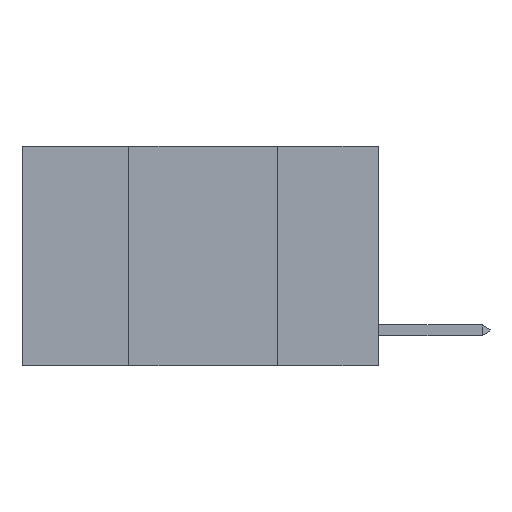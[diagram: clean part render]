
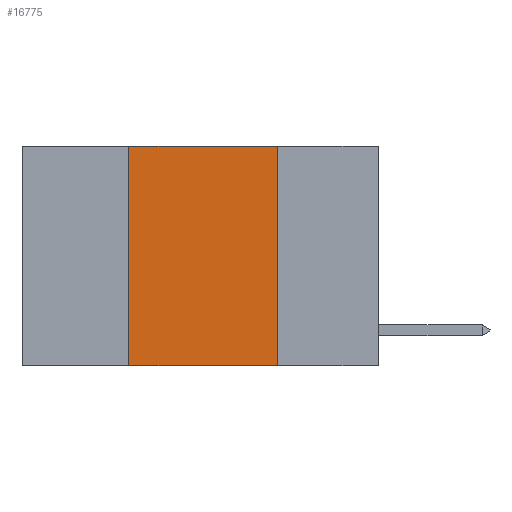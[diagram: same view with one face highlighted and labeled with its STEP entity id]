
A CAD part, left-side view. The second image highlights one B-rep face of the part: STEP entity #16775.
In plain terms, the highlighted planar face has unit normal (-1, 0, 0).
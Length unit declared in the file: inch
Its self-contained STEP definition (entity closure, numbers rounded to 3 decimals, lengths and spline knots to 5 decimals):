
#320 = ORIENTED_EDGE ( 'NONE', *, *, #9972, .T. ) ;
#625 = EDGE_CURVE ( 'NONE', #6422, #5239, #4161, .T. ) ;
#1381 = EDGE_CURVE ( 'NONE', #10255, #18290, #10004, .T. ) ;
#1623 = PLANE ( 'NONE',  #4414 ) ;
#2044 = DIRECTION ( 'NONE',  ( 0., -1., 0. ) ) ;
#2217 = CARTESIAN_POINT ( 'NONE',  ( 0., 0.17, 0. ) ) ;
#3463 = CARTESIAN_POINT ( 'NONE',  ( 0., 0.17, -0.37 ) ) ;
#3628 = CARTESIAN_POINT ( 'NONE',  ( 0., 0.6, -0.37 ) ) ;
#3800 = LINE ( 'NONE', #19191, #20383 ) ;
#4077 = ORIENTED_EDGE ( 'NONE', *, *, #1381, .F. ) ;
#4161 = LINE ( 'NONE', #2217, #12407 ) ;
#4414 = AXIS2_PLACEMENT_3D ( 'NONE', #5006, #17934, #8306 ) ;
#5006 = CARTESIAN_POINT ( 'NONE',  ( 0., 0.6, 0. ) ) ;
#5239 = VERTEX_POINT ( 'NONE', #3463 ) ;
#5644 = VECTOR ( 'NONE', #5695, 39.37008 ) ;
#5695 = DIRECTION ( 'NONE',  ( 0., 0., 1. ) ) ;
#6422 = VERTEX_POINT ( 'NONE', #20838 ) ;
#7595 = ORIENTED_EDGE ( 'NONE', *, *, #7707, .F. ) ;
#7707 = EDGE_CURVE ( 'NONE', #18290, #6422, #3800, .T. ) ;
#8306 = DIRECTION ( 'NONE',  ( 0., 0., -1. ) ) ;
#9619 = DIRECTION ( 'NONE',  ( 0., -1., 0. ) ) ;
#9972 = EDGE_CURVE ( 'NONE', #10255, #5239, #12493, .T. ) ;
#10004 = LINE ( 'NONE', #20072, #5644 ) ;
#10255 = VERTEX_POINT ( 'NONE', #12597 ) ;
#12075 = DIRECTION ( 'NONE',  ( 0., 0., -1. ) ) ;
#12407 = VECTOR ( 'NONE', #12075, 39.37008 ) ;
#12493 = LINE ( 'NONE', #3628, #20337 ) ;
#12597 = CARTESIAN_POINT ( 'NONE',  ( 0., 0.42, -0.37 ) ) ;
#13027 = ORIENTED_EDGE ( 'NONE', *, *, #625, .F. ) ;
#13598 = EDGE_LOOP ( 'NONE', ( #13027, #7595, #4077, #320 ) ) ;
#13665 = FACE_OUTER_BOUND ( 'NONE', #13598, .T. ) ;
#16564 = CARTESIAN_POINT ( 'NONE',  ( 0., 0.42, 0. ) ) ;
#16775 = ADVANCED_FACE ( 'NONE', ( #13665 ), #1623, .F. ) ;
#17934 = DIRECTION ( 'NONE',  ( 1., 0., 0. ) ) ;
#18290 = VERTEX_POINT ( 'NONE', #16564 ) ;
#19191 = CARTESIAN_POINT ( 'NONE',  ( 0., 0.6, 0. ) ) ;
#20072 = CARTESIAN_POINT ( 'NONE',  ( 0., 0.42, 0. ) ) ;
#20337 = VECTOR ( 'NONE', #2044, 39.37008 ) ;
#20383 = VECTOR ( 'NONE', #9619, 39.37008 ) ;
#20838 = CARTESIAN_POINT ( 'NONE',  ( 0., 0.17, 0. ) ) ;
